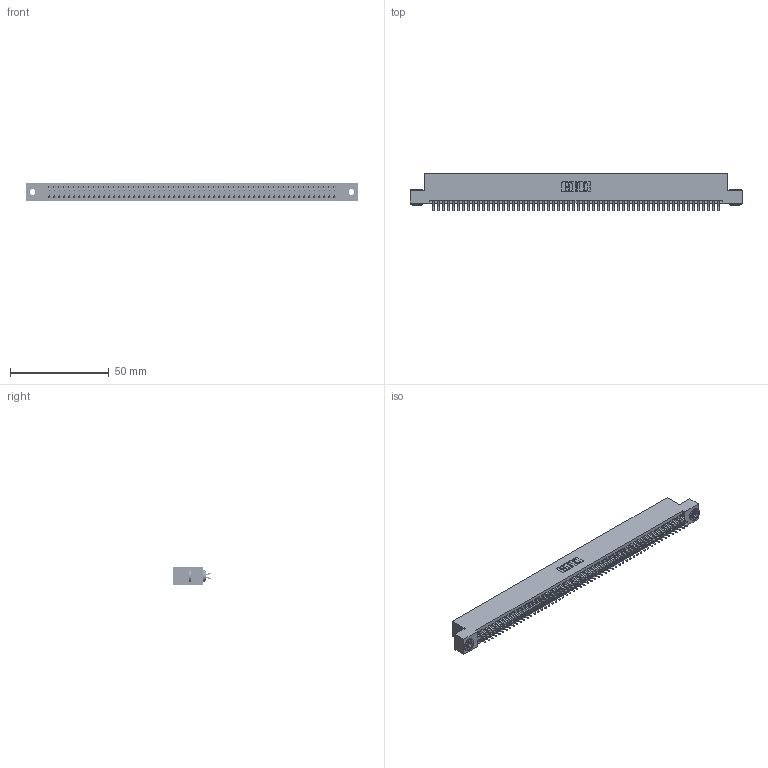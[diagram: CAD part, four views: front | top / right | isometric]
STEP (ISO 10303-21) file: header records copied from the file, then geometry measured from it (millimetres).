
FILE_DESCRIPTION (( 'STEP AP203' ), '1' );
FILE_NAME ('395-116-556-203.STEP', '2018-12-02T02:02:30', ( '' ), ( '' ), 'SwSTEP 2.0', 'SolidWorks 2016', '' );
FILE_SCHEMA (( 'CONFIG_CONTROL_DESIGN' ));
Length unit declared in the file: inch
Products named in the file (4): 395-116-556-203; 345-292-001_556 Tail; 345-250-002_345-250-002-102; 345 Part_Flush Mounting Lugs - 0.156 Dia-TH
Assembly tree (119 placements, depth 2):
  395-116-556-203
    345 Part_Flush Mounting Lugs - 0.156 Dia-TH
    345-292-001_556 Tail  x116
    345-250-002_345-250-002-102  x2
Bounding box: 168.53 x 19.24 x 9.4 mm (x, y, z)
Volume: 16534.4 mm3; surface area: 24853.9 mm2
Topology: 119 solids, 119 shells, 6660 faces, 19789 edges, 13034 vertices
Faces by surface type: plane 4382, cylinder 2270, cone 8
Entity records: 44224 total; most frequent: CARTESIAN_POINT 7387, ORIENTED_EDGE 7302, DIRECTION 6513, EDGE_CURVE 3651, LINE 3255, VECTOR 3255, VERTEX_POINT 2430, AXIS2_PLACEMENT_3D 1629
